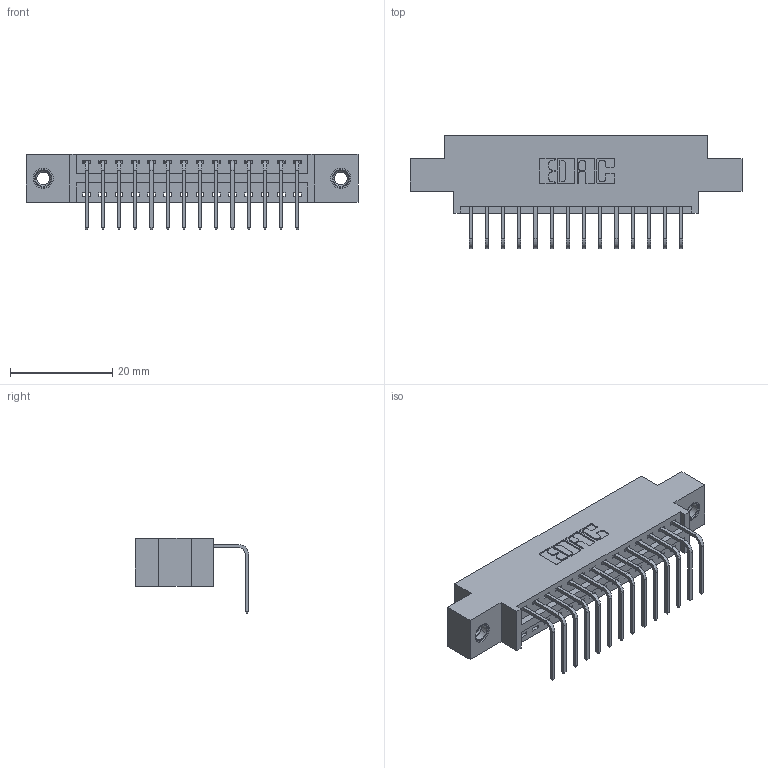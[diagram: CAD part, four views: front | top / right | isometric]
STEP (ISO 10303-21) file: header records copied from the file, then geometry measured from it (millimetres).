
FILE_DESCRIPTION (( 'STEP AP203' ), '1' );
FILE_NAME ('396-014-558-607.STEP', '2019-11-01T05:44:23', ( '' ), ( '' ), 'SwSTEP 2.0', 'SolidWorks 2016', '' );
FILE_SCHEMA (( 'CONFIG_CONTROL_DESIGN' ));
Length unit declared in the file: inch
Products named in the file (4): 345-250-001_345-250-005-103; 396-014-558-607; 346 Part_0.170 Offset - 0.156 Dia-TI; 345-292-001_558 Tail - 2
Assembly tree (17 placements, depth 2):
  396-014-558-607
    346 Part_0.170 Offset - 0.156 Dia-TI
    345-292-001_558 Tail - 2  x14
    345-250-001_345-250-005-103  x2
Bounding box: 65.02 x 22.16 x 14.73 mm (x, y, z)
Volume: 5909.8 mm3; surface area: 7557.6 mm2
Topology: 17 solids, 17 shells, 1026 faces, 3025 edges, 1990 vertices
Faces by surface type: plane 700, cylinder 310, cone 12, torus 4
Entity records: 13860 total; most frequent: CARTESIAN_POINT 2369, ORIENTED_EDGE 2310, DIRECTION 2149, EDGE_CURVE 1155, VECTOR 947, LINE 947, VERTEX_POINT 764, AXIS2_PLACEMENT_3D 601
